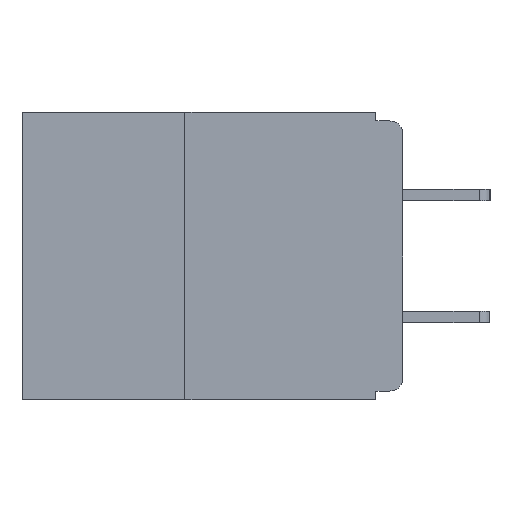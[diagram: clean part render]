
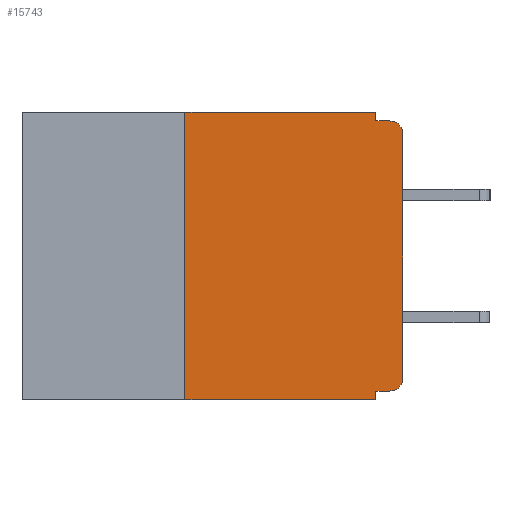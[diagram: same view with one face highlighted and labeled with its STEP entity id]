
A CAD part, left-side view. The second image highlights one B-rep face of the part: STEP entity #15743.
In plain terms, the highlighted planar face has unit normal (-1, 0, 0).
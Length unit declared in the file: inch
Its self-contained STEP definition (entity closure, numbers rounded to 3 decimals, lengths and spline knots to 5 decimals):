
#469 = VECTOR ( 'NONE', #16877, 39.37008 ) ;
#641 = DIRECTION ( 'NONE',  ( 0., -1., 0. ) ) ;
#708 = VECTOR ( 'NONE', #16175, 39.37008 ) ;
#1146 = DIRECTION ( 'NONE',  ( 0., 0., -1. ) ) ;
#1341 = CARTESIAN_POINT ( 'NONE',  ( 0., 0.015, -0.025 ) ) ;
#1903 = CARTESIAN_POINT ( 'NONE',  ( 0., 0., -0.305 ) ) ;
#2218 = CARTESIAN_POINT ( 'NONE',  ( 0., 0.25, 0. ) ) ;
#2394 = EDGE_CURVE ( 'NONE', #16429, #12811, #5167, .T. ) ;
#2533 = CARTESIAN_POINT ( 'NONE',  ( 0., 0.25, -0.33 ) ) ;
#2790 = AXIS2_PLACEMENT_3D ( 'NONE', #1341, #17732, #3745 ) ;
#2851 = CARTESIAN_POINT ( 'NONE',  ( 0., 0.437, 0. ) ) ;
#3228 = ORIENTED_EDGE ( 'NONE', *, *, #29224, .F. ) ;
#3380 = ORIENTED_EDGE ( 'NONE', *, *, #24612, .T. ) ;
#3583 = ORIENTED_EDGE ( 'NONE', *, *, #19249, .F. ) ;
#3616 = ORIENTED_EDGE ( 'NONE', *, *, #19884, .T. ) ;
#3707 = ORIENTED_EDGE ( 'NONE', *, *, #2394, .F. ) ;
#3745 = DIRECTION ( 'NONE',  ( 0., 0., -1. ) ) ;
#3874 = VERTEX_POINT ( 'NONE', #22013 ) ;
#4156 = CARTESIAN_POINT ( 'NONE',  ( 0., 0.015, -0.305 ) ) ;
#5167 = LINE ( 'NONE', #7106, #22364 ) ;
#5447 = FACE_OUTER_BOUND ( 'NONE', #12287, .T. ) ;
#5765 = AXIS2_PLACEMENT_3D ( 'NONE', #4156, #20524, #6497 ) ;
#5817 = PLANE ( 'NONE',  #14243 ) ;
#6497 = DIRECTION ( 'NONE',  ( 0., 0., -1. ) ) ;
#6683 = CARTESIAN_POINT ( 'NONE',  ( 0., 0.25, -0.33 ) ) ;
#6695 = EDGE_CURVE ( 'NONE', #18165, #27606, #18452, .T. ) ;
#7099 = DIRECTION ( 'NONE',  ( 0., 1., 0. ) ) ;
#7106 = CARTESIAN_POINT ( 'NONE',  ( 0., 0., -0.32 ) ) ;
#8476 = CARTESIAN_POINT ( 'NONE',  ( 0., 0.015, -0.32 ) ) ;
#8893 = VERTEX_POINT ( 'NONE', #16062 ) ;
#8902 = LINE ( 'NONE', #27552, #14413 ) ;
#9566 = ORIENTED_EDGE ( 'NONE', *, *, #6695, .F. ) ;
#9652 = ORIENTED_EDGE ( 'NONE', *, *, #20201, .F. ) ;
#9740 = ORIENTED_EDGE ( 'NONE', *, *, #14291, .F. ) ;
#11243 = VERTEX_POINT ( 'NONE', #2533 ) ;
#11475 = VERTEX_POINT ( 'NONE', #29519 ) ;
#12287 = EDGE_LOOP ( 'NONE', ( #18772, #3380, #3228, #9652, #9566, #3583, #3616, #9740, #3707, #21824 ) ) ;
#12811 = VERTEX_POINT ( 'NONE', #27706 ) ;
#12840 = CIRCLE ( 'NONE', #5765, 0.015 ) ;
#13874 = CARTESIAN_POINT ( 'NONE',  ( 0., 0.437, -0.33 ) ) ;
#14089 = VERTEX_POINT ( 'NONE', #21174 ) ;
#14243 = AXIS2_PLACEMENT_3D ( 'NONE', #29193, #15273, #1146 ) ;
#14291 = EDGE_CURVE ( 'NONE', #12811, #8893, #28118, .T. ) ;
#14413 = VECTOR ( 'NONE', #25245, 39.37008 ) ;
#15273 = DIRECTION ( 'NONE',  ( 1., 0., 0. ) ) ;
#15743 = ADVANCED_FACE ( 'NONE', ( #5447 ), #5817, .F. ) ;
#15756 = VECTOR ( 'NONE', #26520, 39.37008 ) ;
#16062 = CARTESIAN_POINT ( 'NONE',  ( 0., 0.031, -0.33 ) ) ;
#16175 = DIRECTION ( 'NONE',  ( 0., -1., 0. ) ) ;
#16429 = VERTEX_POINT ( 'NONE', #8476 ) ;
#16856 = LINE ( 'NONE', #19630, #22345 ) ;
#16877 = DIRECTION ( 'NONE',  ( 0., -1., 0. ) ) ;
#17732 = DIRECTION ( 'NONE',  ( -1., 0., 0. ) ) ;
#18165 = VERTEX_POINT ( 'NONE', #2218 ) ;
#18452 = LINE ( 'NONE', #2851, #469 ) ;
#18772 = ORIENTED_EDGE ( 'NONE', *, *, #21573, .T. ) ;
#19249 = EDGE_CURVE ( 'NONE', #11243, #18165, #30058, .T. ) ;
#19630 = CARTESIAN_POINT ( 'NONE',  ( 0., 0.031, 0. ) ) ;
#19837 = VERTEX_POINT ( 'NONE', #1903 ) ;
#19884 = EDGE_CURVE ( 'NONE', #11243, #8893, #26377, .T. ) ;
#20201 = EDGE_CURVE ( 'NONE', #27606, #3874, #16856, .T. ) ;
#20524 = DIRECTION ( 'NONE',  ( -1., 0., 0. ) ) ;
#21174 = CARTESIAN_POINT ( 'NONE',  ( 0., 0.015, -0.01 ) ) ;
#21573 = EDGE_CURVE ( 'NONE', #19837, #11475, #8902, .T. ) ;
#21786 = CARTESIAN_POINT ( 'NONE',  ( 0., 0., -0.01 ) ) ;
#21824 = ORIENTED_EDGE ( 'NONE', *, *, #28196, .T. ) ;
#21967 = DIRECTION ( 'NONE',  ( 0., 0., -1. ) ) ;
#22013 = CARTESIAN_POINT ( 'NONE',  ( 0., 0.031, -0.01 ) ) ;
#22345 = VECTOR ( 'NONE', #21967, 39.37008 ) ;
#22364 = VECTOR ( 'NONE', #7099, 39.37008 ) ;
#23044 = DIRECTION ( 'NONE',  ( 0., 0., 1. ) ) ;
#24192 = CARTESIAN_POINT ( 'NONE',  ( 0., 0.031, -0.33 ) ) ;
#24612 = EDGE_CURVE ( 'NONE', #11475, #14089, #26560, .T. ) ;
#25245 = DIRECTION ( 'NONE',  ( 0., 0., 1. ) ) ;
#25500 = VECTOR ( 'NONE', #641, 39.37008 ) ;
#26229 = LINE ( 'NONE', #21786, #25500 ) ;
#26377 = LINE ( 'NONE', #13874, #708 ) ;
#26520 = DIRECTION ( 'NONE',  ( 0., 0., -1. ) ) ;
#26560 = CIRCLE ( 'NONE', #2790, 0.015 ) ;
#27552 = CARTESIAN_POINT ( 'NONE',  ( 0., 0., 0. ) ) ;
#27606 = VERTEX_POINT ( 'NONE', #29919 ) ;
#27706 = CARTESIAN_POINT ( 'NONE',  ( 0., 0.031, -0.32 ) ) ;
#28118 = LINE ( 'NONE', #24192, #15756 ) ;
#28196 = EDGE_CURVE ( 'NONE', #16429, #19837, #12840, .T. ) ;
#29193 = CARTESIAN_POINT ( 'NONE',  ( 0., 0.437, 0. ) ) ;
#29224 = EDGE_CURVE ( 'NONE', #3874, #14089, #26229, .T. ) ;
#29307 = VECTOR ( 'NONE', #23044, 39.37008 ) ;
#29519 = CARTESIAN_POINT ( 'NONE',  ( 0., 0., -0.025 ) ) ;
#29919 = CARTESIAN_POINT ( 'NONE',  ( 0., 0.031, 0. ) ) ;
#30058 = LINE ( 'NONE', #6683, #29307 ) ;
